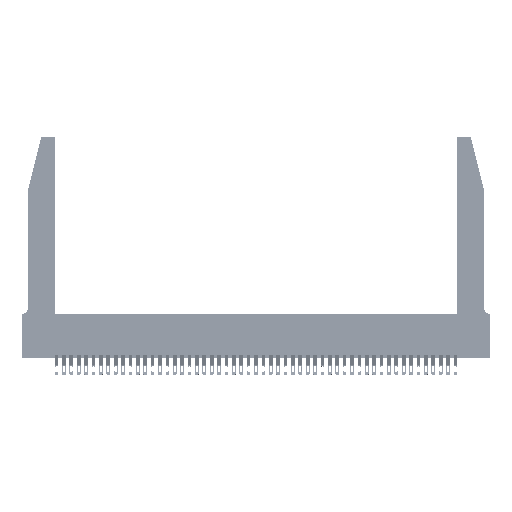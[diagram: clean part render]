
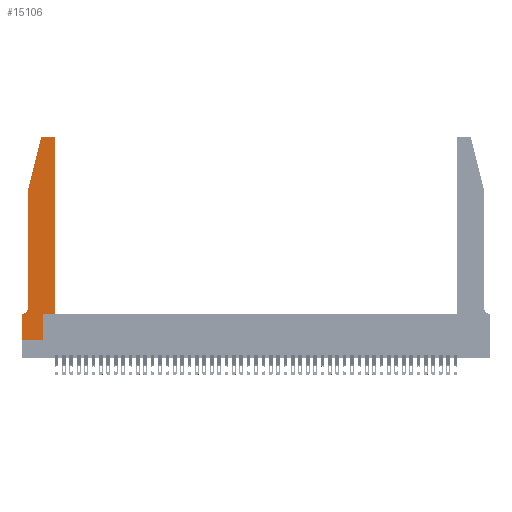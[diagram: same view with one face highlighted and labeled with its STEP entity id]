
A CAD part, top view. The second image highlights one B-rep face of the part: STEP entity #15106.
In plain terms, the highlighted planar face has unit normal (0, 0, 1).
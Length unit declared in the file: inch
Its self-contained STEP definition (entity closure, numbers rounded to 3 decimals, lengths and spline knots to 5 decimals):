
#373 = CARTESIAN_POINT ( 'NONE',  ( 0.2865, 0.35, 0.37 ) ) ;
#763 = CIRCLE ( 'NONE', #25582, 0.03 ) ;
#1002 = CARTESIAN_POINT ( 'NONE',  ( 0.4505, 0.35, 0.37 ) ) ;
#1080 = DIRECTION ( 'NONE',  ( 1., 0., 0. ) ) ;
#2237 = VERTEX_POINT ( 'NONE', #8720 ) ;
#2399 = VERTEX_POINT ( 'NONE', #31462 ) ;
#2977 = EDGE_CURVE ( 'NONE', #2237, #26691, #24226, .T. ) ;
#3506 = DIRECTION ( 'NONE',  ( 0., 0., 1. ) ) ;
#3751 = DIRECTION ( 'NONE',  ( 1., 0., 0. ) ) ;
#3955 = EDGE_LOOP ( 'NONE', ( #17629, #44491, #32715, #13118, #10249, #33764, #41731, #5204, #33802, #12491, #37073, #13555 ) ) ;
#4343 = LINE ( 'NONE', #31699, #31885 ) ;
#5135 = VECTOR ( 'NONE', #17033, 39.37008 ) ;
#5204 = ORIENTED_EDGE ( 'NONE', *, *, #25135, .T. ) ;
#5986 = AXIS2_PLACEMENT_3D ( 'NONE', #40196, #18757, #43808 ) ;
#6126 = AXIS2_PLACEMENT_3D ( 'NONE', #25032, #3506, #28638 ) ;
#6172 = CARTESIAN_POINT ( 'NONE',  ( 0., 0., 0.37 ) ) ;
#6394 = VERTEX_POINT ( 'NONE', #17800 ) ;
#6898 = CARTESIAN_POINT ( 'NONE',  ( 0.2865, 0.35, 0.37 ) ) ;
#7935 = VECTOR ( 'NONE', #36935, 39.37008 ) ;
#8720 = CARTESIAN_POINT ( 'NONE',  ( 0.2865, 0., 0.37 ) ) ;
#8938 = EDGE_CURVE ( 'NONE', #17442, #9914, #763, .T. ) ;
#9716 = VECTOR ( 'NONE', #13982, 39.37008 ) ;
#9914 = VERTEX_POINT ( 'NONE', #43379 ) ;
#10249 = ORIENTED_EDGE ( 'NONE', *, *, #38481, .T. ) ;
#10904 = CARTESIAN_POINT ( 'NONE',  ( 0., 0.35, 0.37 ) ) ;
#11911 = VECTOR ( 'NONE', #39385, 39.37008 ) ;
#12491 = ORIENTED_EDGE ( 'NONE', *, *, #13236, .T. ) ;
#13118 = ORIENTED_EDGE ( 'NONE', *, *, #36946, .T. ) ;
#13236 = EDGE_CURVE ( 'NONE', #26691, #2399, #27465, .T. ) ;
#13555 = ORIENTED_EDGE ( 'NONE', *, *, #20196, .T. ) ;
#13982 = DIRECTION ( 'NONE',  ( -1., 0., 0. ) ) ;
#14514 = CARTESIAN_POINT ( 'NONE',  ( 0.0055, 0.35, 0.37 ) ) ;
#14714 = VECTOR ( 'NONE', #25098, 39.37008 ) ;
#14740 = CARTESIAN_POINT ( 'NONE',  ( 0., 0., 0.37 ) ) ;
#15106 = ADVANCED_FACE ( 'NONE', ( #30161 ), #21720, .T. ) ;
#16205 = CARTESIAN_POINT ( 'NONE',  ( 0.284, 2.72, 0.37 ) ) ;
#16945 = CARTESIAN_POINT ( 'NONE',  ( 0.0755, 2., 0.37 ) ) ;
#17032 = LINE ( 'NONE', #14740, #25417 ) ;
#17033 = DIRECTION ( 'NONE',  ( 1., 0., 0. ) ) ;
#17442 = VERTEX_POINT ( 'NONE', #37953 ) ;
#17629 = ORIENTED_EDGE ( 'NONE', *, *, #17639, .T. ) ;
#17639 = EDGE_CURVE ( 'NONE', #32386, #17442, #19280, .T. ) ;
#17800 = CARTESIAN_POINT ( 'NONE',  ( 0., 0.35, 0.37 ) ) ;
#18042 = VERTEX_POINT ( 'NONE', #24290 ) ;
#18402 = EDGE_CURVE ( 'NONE', #2399, #31517, #43862, .T. ) ;
#18757 = DIRECTION ( 'NONE',  ( 0., 0., -1. ) ) ;
#19280 = LINE ( 'NONE', #39035, #9716 ) ;
#19812 = DIRECTION ( 'NONE',  ( 1., 0., 0. ) ) ;
#20196 = EDGE_CURVE ( 'NONE', #31517, #32386, #42662, .T. ) ;
#21720 = PLANE ( 'NONE',  #28248 ) ;
#22566 = LINE ( 'NONE', #28552, #11911 ) ;
#24226 = LINE ( 'NONE', #6898, #14714 ) ;
#24247 = LINE ( 'NONE', #6172, #5135 ) ;
#24290 = CARTESIAN_POINT ( 'NONE',  ( 0., 0., 0.37 ) ) ;
#25032 = CARTESIAN_POINT ( 'NONE',  ( 0.4205, 2.72, 0.37 ) ) ;
#25098 = DIRECTION ( 'NONE',  ( 0., 1., 0. ) ) ;
#25135 = EDGE_CURVE ( 'NONE', #18042, #2237, #24247, .T. ) ;
#25281 = DIRECTION ( 'NONE',  ( 0., 0., 1. ) ) ;
#25417 = VECTOR ( 'NONE', #36179, 39.37008 ) ;
#25582 = AXIS2_PLACEMENT_3D ( 'NONE', #16205, #41255, #19812 ) ;
#26346 = VECTOR ( 'NONE', #1080, 39.37008 ) ;
#26691 = VERTEX_POINT ( 'NONE', #373 ) ;
#27465 = LINE ( 'NONE', #40495, #26346 ) ;
#28248 = AXIS2_PLACEMENT_3D ( 'NONE', #10904, #25281, #3751 ) ;
#28552 = CARTESIAN_POINT ( 'NONE',  ( 0.0755, 2., 0.37 ) ) ;
#28638 = DIRECTION ( 'NONE',  ( 1., 0., 0. ) ) ;
#30161 = FACE_OUTER_BOUND ( 'NONE', #3955, .T. ) ;
#30205 = CARTESIAN_POINT ( 'NONE',  ( 0.0755, 2., 0.37 ) ) ;
#31445 = CARTESIAN_POINT ( 'NONE',  ( 0.4205, 2.75, 0.37 ) ) ;
#31462 = CARTESIAN_POINT ( 'NONE',  ( 0.4505, 0.35, 0.37 ) ) ;
#31517 = VERTEX_POINT ( 'NONE', #37301 ) ;
#31699 = CARTESIAN_POINT ( 'NONE',  ( 0.0755, 0.35, 0.37 ) ) ;
#31885 = VECTOR ( 'NONE', #35284, 39.37008 ) ;
#32386 = VERTEX_POINT ( 'NONE', #31445 ) ;
#32603 = VERTEX_POINT ( 'NONE', #14514 ) ;
#32678 = VERTEX_POINT ( 'NONE', #36404 ) ;
#32715 = ORIENTED_EDGE ( 'NONE', *, *, #37517, .T. ) ;
#33068 = VERTEX_POINT ( 'NONE', #30205 ) ;
#33764 = ORIENTED_EDGE ( 'NONE', *, *, #38818, .T. ) ;
#33802 = ORIENTED_EDGE ( 'NONE', *, *, #2977, .T. ) ;
#34939 = DIRECTION ( 'NONE',  ( -0.239, -0.971, 0. ) ) ;
#35284 = DIRECTION ( 'NONE',  ( -1., 0., 0. ) ) ;
#36179 = DIRECTION ( 'NONE',  ( 0., -1., 0. ) ) ;
#36404 = CARTESIAN_POINT ( 'NONE',  ( 0.0755, 0.42, 0.37 ) ) ;
#36935 = DIRECTION ( 'NONE',  ( 0., 1., 0. ) ) ;
#36946 = EDGE_CURVE ( 'NONE', #33068, #32678, #22566, .T. ) ;
#37048 = VECTOR ( 'NONE', #34939, 39.37008 ) ;
#37073 = ORIENTED_EDGE ( 'NONE', *, *, #18402, .T. ) ;
#37301 = CARTESIAN_POINT ( 'NONE',  ( 0.4505, 2.72, 0.37 ) ) ;
#37517 = EDGE_CURVE ( 'NONE', #9914, #33068, #38183, .T. ) ;
#37953 = CARTESIAN_POINT ( 'NONE',  ( 0.284, 2.75, 0.37 ) ) ;
#38183 = LINE ( 'NONE', #16945, #37048 ) ;
#38481 = EDGE_CURVE ( 'NONE', #32678, #32603, #45383, .T. ) ;
#38818 = EDGE_CURVE ( 'NONE', #32603, #6394, #4343, .T. ) ;
#39035 = CARTESIAN_POINT ( 'NONE',  ( 0.2605, 2.75, 0.37 ) ) ;
#39385 = DIRECTION ( 'NONE',  ( 0., -1., 0. ) ) ;
#40196 = CARTESIAN_POINT ( 'NONE',  ( 0.0055, 0.42, 0.37 ) ) ;
#40495 = CARTESIAN_POINT ( 'NONE',  ( 0.4505, 0.35, 0.37 ) ) ;
#41255 = DIRECTION ( 'NONE',  ( 0., 0., 1. ) ) ;
#41731 = ORIENTED_EDGE ( 'NONE', *, *, #42626, .T. ) ;
#42626 = EDGE_CURVE ( 'NONE', #6394, #18042, #17032, .T. ) ;
#42662 = CIRCLE ( 'NONE', #6126, 0.03 ) ;
#43379 = CARTESIAN_POINT ( 'NONE',  ( 0.25487, 2.72718, 0.37 ) ) ;
#43808 = DIRECTION ( 'NONE',  ( -1., 0., 0. ) ) ;
#43862 = LINE ( 'NONE', #1002, #7935 ) ;
#44491 = ORIENTED_EDGE ( 'NONE', *, *, #8938, .T. ) ;
#45383 = CIRCLE ( 'NONE', #5986, 0.07 ) ;
